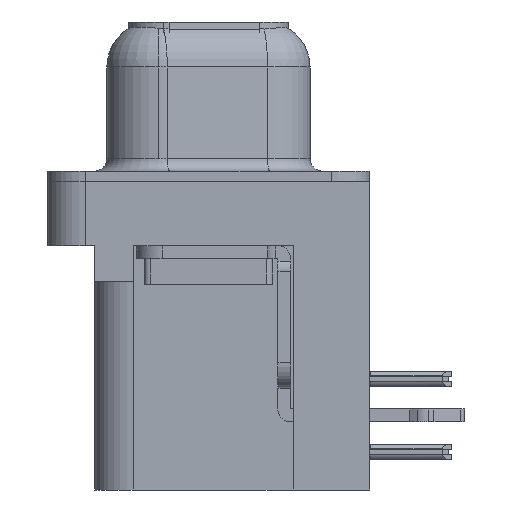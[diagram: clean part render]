
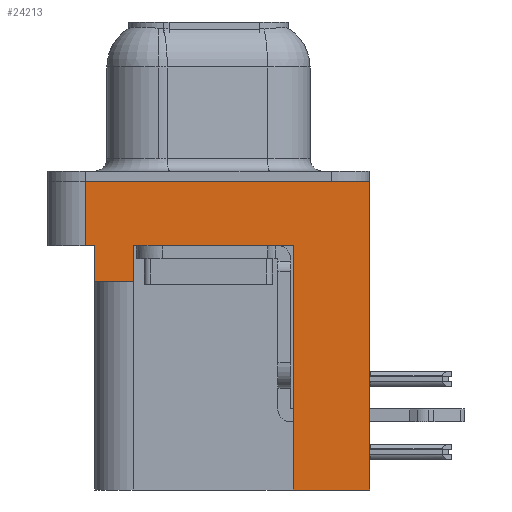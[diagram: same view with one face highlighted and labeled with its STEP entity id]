
A CAD part, left-side view. The second image highlights one B-rep face of the part: STEP entity #24213.
In plain terms, the highlighted planar face has unit normal (-1, 0, 0).
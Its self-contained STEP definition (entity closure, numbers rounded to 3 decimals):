
#100 = VECTOR ( 'NONE', #24127, 1000. ) ;
#250 = EDGE_CURVE ( 'NONE', #16502, #25841, #18438, .T. ) ;
#624 = EDGE_LOOP ( 'NONE', ( #9597, #29475, #8289, #2066, #2346, #23374, #16443, #29629, #11871, #22095 ) ) ;
#997 = EDGE_CURVE ( 'NONE', #16502, #8328, #17461, .T. ) ;
#1675 = EDGE_CURVE ( 'NONE', #14899, #15367, #18187, .T. ) ;
#1887 = CARTESIAN_POINT ( 'NONE',  ( -3., -3.295, -12. ) ) ;
#2066 = ORIENTED_EDGE ( 'NONE', *, *, #1675, .F. ) ;
#2346 = ORIENTED_EDGE ( 'NONE', *, *, #3440, .F. ) ;
#3407 = CARTESIAN_POINT ( 'NONE',  ( -3., -6.275, 0. ) ) ;
#3440 = EDGE_CURVE ( 'NONE', #28733, #14899, #29670, .T. ) ;
#3909 = VERTEX_POINT ( 'NONE', #10345 ) ;
#4267 = EDGE_CURVE ( 'NONE', #25950, #8328, #16785, .T. ) ;
#4608 = AXIS2_PLACEMENT_3D ( 'NONE', #12917, #27590, #15574 ) ;
#5774 = CARTESIAN_POINT ( 'NONE',  ( -3., -3.295, -12. ) ) ;
#5968 = VECTOR ( 'NONE', #13017, 1000. ) ;
#5991 = CARTESIAN_POINT ( 'NONE',  ( -3., 4.425, -3.9 ) ) ;
#6483 = VECTOR ( 'NONE', #18283, 1000. ) ;
#7285 = CARTESIAN_POINT ( 'NONE',  ( -3., -3.295, -12. ) ) ;
#7404 = CARTESIAN_POINT ( 'NONE',  ( -3., 2.895, -3.9 ) ) ;
#7683 = EDGE_CURVE ( 'NONE', #25841, #3909, #14950, .T. ) ;
#7816 = VECTOR ( 'NONE', #26430, 1000. ) ;
#8289 = ORIENTED_EDGE ( 'NONE', *, *, #19515, .T. ) ;
#8328 = VERTEX_POINT ( 'NONE', #3407 ) ;
#8467 = VECTOR ( 'NONE', #9136, 1000. ) ;
#8470 = CARTESIAN_POINT ( 'NONE',  ( -3., 4.775, -2.5 ) ) ;
#9136 = DIRECTION ( 'NONE',  ( 0., 0., 1. ) ) ;
#9168 = CARTESIAN_POINT ( 'NONE',  ( -3., 4.775, 0. ) ) ;
#9246 = CARTESIAN_POINT ( 'NONE',  ( -3., 4.425, -3.9 ) ) ;
#9597 = ORIENTED_EDGE ( 'NONE', *, *, #4267, .F. ) ;
#9845 = CARTESIAN_POINT ( 'NONE',  ( -3., -6.275, 0. ) ) ;
#10345 = CARTESIAN_POINT ( 'NONE',  ( -3., -3.295, -2.5 ) ) ;
#11871 = ORIENTED_EDGE ( 'NONE', *, *, #250, .F. ) ;
#11885 = CARTESIAN_POINT ( 'NONE',  ( -3., -6.275, -12. ) ) ;
#12304 = DIRECTION ( 'NONE',  ( 0., -1., 0. ) ) ;
#12917 = CARTESIAN_POINT ( 'NONE',  ( -3., -6.275, -2.5 ) ) ;
#13006 = LINE ( 'NONE', #21492, #100 ) ;
#13017 = DIRECTION ( 'NONE',  ( 0., 0., 1. ) ) ;
#13732 = VERTEX_POINT ( 'NONE', #8470 ) ;
#13792 = VECTOR ( 'NONE', #22093, 1000. ) ;
#14899 = VERTEX_POINT ( 'NONE', #5991 ) ;
#14950 = LINE ( 'NONE', #1887, #8467 ) ;
#15367 = VERTEX_POINT ( 'NONE', #25679 ) ;
#15545 = DIRECTION ( 'NONE',  ( 0., 1., 0. ) ) ;
#15574 = DIRECTION ( 'NONE',  ( 0., 0., 1. ) ) ;
#16443 = ORIENTED_EDGE ( 'NONE', *, *, #22415, .T. ) ;
#16502 = VERTEX_POINT ( 'NONE', #11885 ) ;
#16663 = LINE ( 'NONE', #22003, #27643 ) ;
#16785 = LINE ( 'NONE', #9845, #30385 ) ;
#17461 = LINE ( 'NONE', #18504, #6483 ) ;
#17980 = PLANE ( 'NONE',  #4608 ) ;
#18074 = EDGE_CURVE ( 'NONE', #13732, #25950, #24884, .T. ) ;
#18085 = FACE_OUTER_BOUND ( 'NONE', #624, .T. ) ;
#18187 = LINE ( 'NONE', #9246, #29517 ) ;
#18283 = DIRECTION ( 'NONE',  ( 0., 0., 1. ) ) ;
#18438 = LINE ( 'NONE', #7285, #7816 ) ;
#18504 = CARTESIAN_POINT ( 'NONE',  ( -3., -6.275, -2.5 ) ) ;
#18730 = DIRECTION ( 'NONE',  ( 0., 0., 1. ) ) ;
#19515 = EDGE_CURVE ( 'NONE', #13732, #15367, #13006, .T. ) ;
#20326 = VERTEX_POINT ( 'NONE', #31055 ) ;
#20974 = LINE ( 'NONE', #7404, #13792 ) ;
#21492 = CARTESIAN_POINT ( 'NONE',  ( -3., -6.275, -2.5 ) ) ;
#22003 = CARTESIAN_POINT ( 'NONE',  ( -3., -6.275, -2.5 ) ) ;
#22093 = DIRECTION ( 'NONE',  ( 0., 0., 1. ) ) ;
#22095 = ORIENTED_EDGE ( 'NONE', *, *, #997, .T. ) ;
#22415 = EDGE_CURVE ( 'NONE', #20326, #3909, #16663, .T. ) ;
#23330 = CARTESIAN_POINT ( 'NONE',  ( -3., 2.895, -3.9 ) ) ;
#23374 = ORIENTED_EDGE ( 'NONE', *, *, #24851, .T. ) ;
#24127 = DIRECTION ( 'NONE',  ( 0., -1., 0. ) ) ;
#24213 = ADVANCED_FACE ( 'NONE', ( #18085 ), #17980, .T. ) ;
#24847 = CARTESIAN_POINT ( 'NONE',  ( -3., 4.775, -2.5 ) ) ;
#24851 = EDGE_CURVE ( 'NONE', #28733, #20326, #20974, .T. ) ;
#24884 = LINE ( 'NONE', #24847, #5968 ) ;
#25679 = CARTESIAN_POINT ( 'NONE',  ( -3., 4.425, -2.5 ) ) ;
#25841 = VERTEX_POINT ( 'NONE', #5774 ) ;
#25950 = VERTEX_POINT ( 'NONE', #9168 ) ;
#26430 = DIRECTION ( 'NONE',  ( 0., 1., 0. ) ) ;
#26910 = CARTESIAN_POINT ( 'NONE',  ( -3., 4.425, -3.9 ) ) ;
#27391 = DIRECTION ( 'NONE',  ( 0., -1., 0. ) ) ;
#27590 = DIRECTION ( 'NONE',  ( -1., 0., 0. ) ) ;
#27643 = VECTOR ( 'NONE', #27391, 1000. ) ;
#28733 = VERTEX_POINT ( 'NONE', #23330 ) ;
#29475 = ORIENTED_EDGE ( 'NONE', *, *, #18074, .F. ) ;
#29517 = VECTOR ( 'NONE', #18730, 1000. ) ;
#29629 = ORIENTED_EDGE ( 'NONE', *, *, #7683, .F. ) ;
#29670 = LINE ( 'NONE', #26910, #30075 ) ;
#30075 = VECTOR ( 'NONE', #15545, 1000. ) ;
#30385 = VECTOR ( 'NONE', #12304, 1000. ) ;
#31055 = CARTESIAN_POINT ( 'NONE',  ( -3., 2.895, -2.5 ) ) ;
